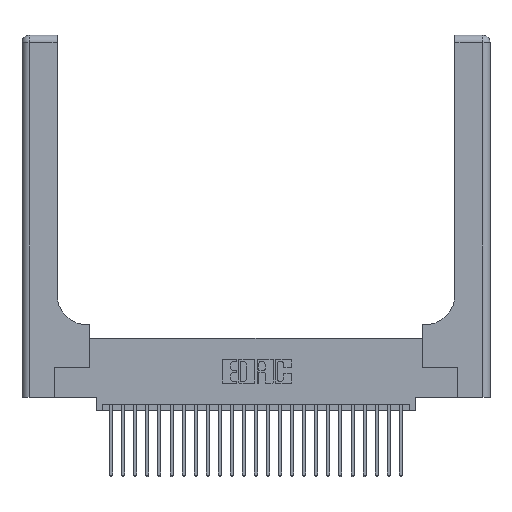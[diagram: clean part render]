
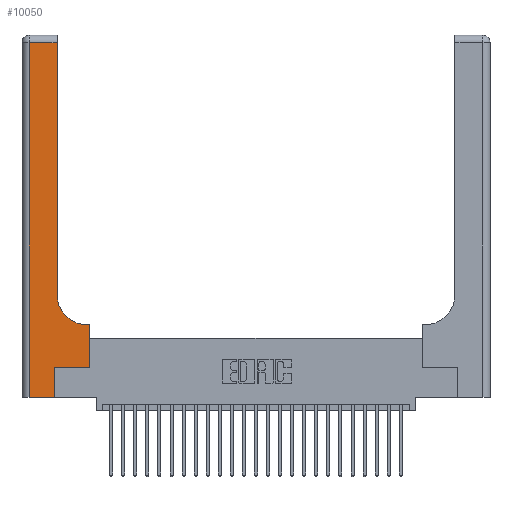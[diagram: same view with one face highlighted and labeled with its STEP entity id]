
A CAD part, top view. The second image highlights one B-rep face of the part: STEP entity #10050.
In plain terms, the highlighted planar face has unit normal (0, 0, 1).
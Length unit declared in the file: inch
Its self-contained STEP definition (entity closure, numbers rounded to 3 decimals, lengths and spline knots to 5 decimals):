
#461 = CARTESIAN_POINT ( 'NONE',  ( 0.269, 0.25, 0.37 ) ) ;
#901 = LINE ( 'NONE', #8313, #16068 ) ;
#1226 = VECTOR ( 'NONE', #14566, 39.37008 ) ;
#1539 = AXIS2_PLACEMENT_3D ( 'NONE', #8037, #16616, #10177 ) ;
#1673 = ORIENTED_EDGE ( 'NONE', *, *, #16834, .T. ) ;
#1761 = AXIS2_PLACEMENT_3D ( 'NONE', #14579, #1978, #14387 ) ;
#1819 = CARTESIAN_POINT ( 'NONE',  ( 0., 0., 0.37 ) ) ;
#1978 = DIRECTION ( 'NONE',  ( 0., 0., -1. ) ) ;
#3105 = CIRCLE ( 'NONE', #1539, 0.25 ) ;
#3202 = DIRECTION ( 'NONE',  ( 1., 0., 0. ) ) ;
#3428 = CARTESIAN_POINT ( 'NONE',  ( 0.06, 0., 0.37 ) ) ;
#3556 = LINE ( 'NONE', #20903, #1226 ) ;
#4034 = VERTEX_POINT ( 'NONE', #19267 ) ;
#4225 = CARTESIAN_POINT ( 'NONE',  ( 0.06, 3., 0.37 ) ) ;
#4886 = VECTOR ( 'NONE', #21696, 39.37008 ) ;
#5883 = VECTOR ( 'NONE', #21764, 39.37008 ) ;
#6429 = EDGE_CURVE ( 'NONE', #20003, #14136, #15543, .T. ) ;
#7341 = VERTEX_POINT ( 'NONE', #24239 ) ;
#7372 = DIRECTION ( 'NONE',  ( 0., -1., 0. ) ) ;
#8037 = CARTESIAN_POINT ( 'NONE',  ( 0.5415, 0.85, 0.37 ) ) ;
#8089 = CARTESIAN_POINT ( 'NONE',  ( 0.5585, 0.25, 0.37 ) ) ;
#8313 = CARTESIAN_POINT ( 'NONE',  ( 0.269, 0., 0.37 ) ) ;
#8348 = VERTEX_POINT ( 'NONE', #12090 ) ;
#9466 = VECTOR ( 'NONE', #12105, 39.37008 ) ;
#9682 = CARTESIAN_POINT ( 'NONE',  ( 0.269, 0.25, 0.37 ) ) ;
#9900 = VECTOR ( 'NONE', #7372, 39.37008 ) ;
#10050 = ADVANCED_FACE ( 'NONE', ( #14115 ), #12531, .F. ) ;
#10177 = DIRECTION ( 'NONE',  ( 1., 0., 0. ) ) ;
#10259 = CARTESIAN_POINT ( 'NONE',  ( 0.5585, 0.25, 0.37 ) ) ;
#10455 = DIRECTION ( 'NONE',  ( 0., 1., 0. ) ) ;
#10850 = ORIENTED_EDGE ( 'NONE', *, *, #6429, .T. ) ;
#12090 = CARTESIAN_POINT ( 'NONE',  ( 0.5415, 0.6, 0.37 ) ) ;
#12105 = DIRECTION ( 'NONE',  ( 1., 0., 0. ) ) ;
#12320 = VECTOR ( 'NONE', #3202, 39.37008 ) ;
#12531 = PLANE ( 'NONE',  #1761 ) ;
#12537 = VECTOR ( 'NONE', #18692, 39.37008 ) ;
#14115 = FACE_OUTER_BOUND ( 'NONE', #18693, .T. ) ;
#14136 = VERTEX_POINT ( 'NONE', #3428 ) ;
#14387 = DIRECTION ( 'NONE',  ( -1., 0., 0. ) ) ;
#14566 = DIRECTION ( 'NONE',  ( 0., 1., 0. ) ) ;
#14579 = CARTESIAN_POINT ( 'NONE',  ( 0., 3., 0.37 ) ) ;
#15474 = EDGE_CURVE ( 'NONE', #25731, #22943, #26043, .T. ) ;
#15543 = LINE ( 'NONE', #4225, #9900 ) ;
#15693 = VERTEX_POINT ( 'NONE', #461 ) ;
#16068 = VECTOR ( 'NONE', #10455, 39.37008 ) ;
#16616 = DIRECTION ( 'NONE',  ( 0., 0., -1. ) ) ;
#16834 = EDGE_CURVE ( 'NONE', #4034, #15693, #901, .T. ) ;
#17089 = EDGE_CURVE ( 'NONE', #22943, #8348, #24934, .T. ) ;
#17090 = LINE ( 'NONE', #26004, #4886 ) ;
#17093 = ORIENTED_EDGE ( 'NONE', *, *, #19586, .T. ) ;
#17457 = EDGE_CURVE ( 'NONE', #21597, #7341, #3556, .T. ) ;
#17708 = ORIENTED_EDGE ( 'NONE', *, *, #24004, .T. ) ;
#17815 = CARTESIAN_POINT ( 'NONE',  ( 0.2915, 0.85, 0.37 ) ) ;
#18692 = DIRECTION ( 'NONE',  ( 0., 1., 0. ) ) ;
#18693 = EDGE_LOOP ( 'NONE', ( #19060, #17708, #10850, #24817, #1673, #22910, #19300, #21926, #17093 ) ) ;
#19060 = ORIENTED_EDGE ( 'NONE', *, *, #17457, .T. ) ;
#19267 = CARTESIAN_POINT ( 'NONE',  ( 0.269, 0., 0.37 ) ) ;
#19300 = ORIENTED_EDGE ( 'NONE', *, *, #15474, .T. ) ;
#19389 = EDGE_CURVE ( 'NONE', #15693, #25731, #20217, .T. ) ;
#19586 = EDGE_CURVE ( 'NONE', #8348, #21597, #3105, .T. ) ;
#20003 = VERTEX_POINT ( 'NONE', #22870 ) ;
#20217 = LINE ( 'NONE', #9682, #12320 ) ;
#20449 = CARTESIAN_POINT ( 'NONE',  ( 0.5585, 0.6, 0.37 ) ) ;
#20903 = CARTESIAN_POINT ( 'NONE',  ( 0.2915, 3., 0.37 ) ) ;
#21573 = CARTESIAN_POINT ( 'NONE',  ( 0.2915, 0.6, 0.37 ) ) ;
#21597 = VERTEX_POINT ( 'NONE', #17815 ) ;
#21696 = DIRECTION ( 'NONE',  ( -1., 0., 0. ) ) ;
#21764 = DIRECTION ( 'NONE',  ( -1., 0., 0. ) ) ;
#21926 = ORIENTED_EDGE ( 'NONE', *, *, #17089, .T. ) ;
#22870 = CARTESIAN_POINT ( 'NONE',  ( 0.06, 2.94, 0.37 ) ) ;
#22910 = ORIENTED_EDGE ( 'NONE', *, *, #19389, .T. ) ;
#22943 = VERTEX_POINT ( 'NONE', #20449 ) ;
#24004 = EDGE_CURVE ( 'NONE', #7341, #20003, #17090, .T. ) ;
#24239 = CARTESIAN_POINT ( 'NONE',  ( 0.2915, 2.94, 0.37 ) ) ;
#24817 = ORIENTED_EDGE ( 'NONE', *, *, #25092, .T. ) ;
#24934 = LINE ( 'NONE', #21573, #5883 ) ;
#24979 = LINE ( 'NONE', #1819, #9466 ) ;
#25092 = EDGE_CURVE ( 'NONE', #14136, #4034, #24979, .T. ) ;
#25731 = VERTEX_POINT ( 'NONE', #10259 ) ;
#26004 = CARTESIAN_POINT ( 'NONE',  ( 0., 2.94, 0.37 ) ) ;
#26043 = LINE ( 'NONE', #8089, #12537 ) ;
